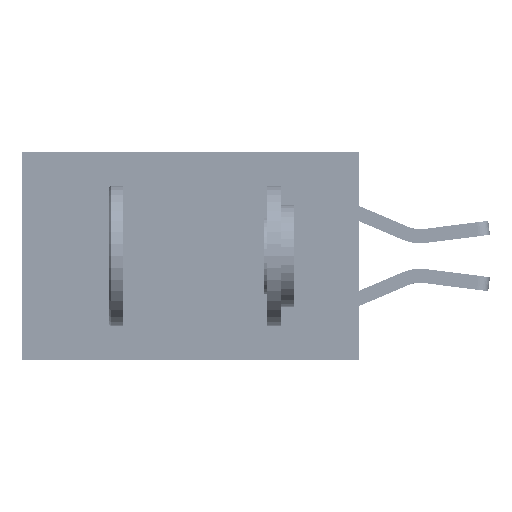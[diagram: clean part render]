
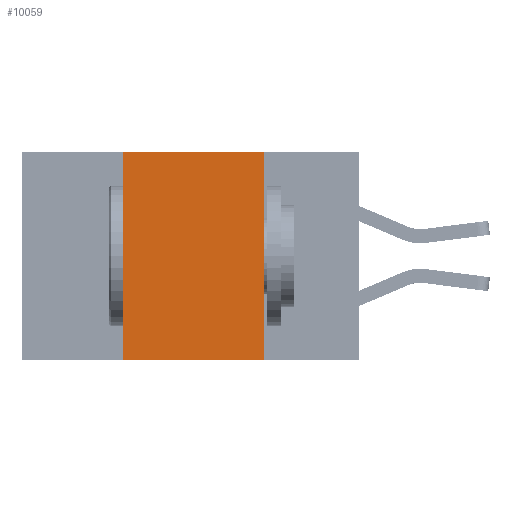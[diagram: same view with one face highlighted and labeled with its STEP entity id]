
A CAD part, left-side view. The second image highlights one B-rep face of the part: STEP entity #10059.
In plain terms, the highlighted planar face has unit normal (-1, 0, 0).
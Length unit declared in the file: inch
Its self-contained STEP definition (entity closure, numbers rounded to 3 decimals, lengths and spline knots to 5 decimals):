
#888 = DIRECTION ( 'NONE',  ( 0., -1., 0. ) ) ;
#1438 = AXIS2_PLACEMENT_3D ( 'NONE', #20532, #17579, #11878 ) ;
#1568 = CARTESIAN_POINT ( 'NONE',  ( 0., 0.17, 0. ) ) ;
#2383 = LINE ( 'NONE', #25675, #35650 ) ;
#6683 = VERTEX_POINT ( 'NONE', #29242 ) ;
#6698 = CARTESIAN_POINT ( 'NONE',  ( 0., 0.17, 0. ) ) ;
#7846 = LINE ( 'NONE', #27850, #27617 ) ;
#10059 = ADVANCED_FACE ( 'NONE', ( #21347 ), #17449, .F. ) ;
#10571 = VECTOR ( 'NONE', #32311, 39.37008 ) ;
#11878 = DIRECTION ( 'NONE',  ( 0., 0., -1. ) ) ;
#11936 = VECTOR ( 'NONE', #23504, 39.37008 ) ;
#13055 = ORIENTED_EDGE ( 'NONE', *, *, #19719, .T. ) ;
#13424 = CARTESIAN_POINT ( 'NONE',  ( 0., 0.6, -0.37 ) ) ;
#17449 = PLANE ( 'NONE',  #1438 ) ;
#17579 = DIRECTION ( 'NONE',  ( 1., 0., 0. ) ) ;
#17670 = ORIENTED_EDGE ( 'NONE', *, *, #34739, .F. ) ;
#18799 = LINE ( 'NONE', #13424, #10571 ) ;
#19719 = EDGE_CURVE ( 'NONE', #39744, #6683, #18799, .T. ) ;
#20236 = EDGE_CURVE ( 'NONE', #22238, #36506, #2383, .T. ) ;
#20532 = CARTESIAN_POINT ( 'NONE',  ( 0., 0.6, 0. ) ) ;
#21257 = ORIENTED_EDGE ( 'NONE', *, *, #36432, .F. ) ;
#21347 = FACE_OUTER_BOUND ( 'NONE', #24152, .T. ) ;
#21725 = ORIENTED_EDGE ( 'NONE', *, *, #20236, .F. ) ;
#22238 = VERTEX_POINT ( 'NONE', #34792 ) ;
#23504 = DIRECTION ( 'NONE',  ( 0., 0., -1. ) ) ;
#24152 = EDGE_LOOP ( 'NONE', ( #17670, #21725, #21257, #13055 ) ) ;
#24487 = DIRECTION ( 'NONE',  ( 0., 0., 1. ) ) ;
#25675 = CARTESIAN_POINT ( 'NONE',  ( 0., 0.6, 0. ) ) ;
#26986 = CARTESIAN_POINT ( 'NONE',  ( 0., 0.42, -0.37 ) ) ;
#27617 = VECTOR ( 'NONE', #24487, 39.37008 ) ;
#27850 = CARTESIAN_POINT ( 'NONE',  ( 0., 0.42, 0. ) ) ;
#29242 = CARTESIAN_POINT ( 'NONE',  ( 0., 0.17, -0.37 ) ) ;
#32311 = DIRECTION ( 'NONE',  ( 0., -1., 0. ) ) ;
#34739 = EDGE_CURVE ( 'NONE', #36506, #6683, #39507, .T. ) ;
#34792 = CARTESIAN_POINT ( 'NONE',  ( 0., 0.42, 0. ) ) ;
#35650 = VECTOR ( 'NONE', #888, 39.37008 ) ;
#36432 = EDGE_CURVE ( 'NONE', #39744, #22238, #7846, .T. ) ;
#36506 = VERTEX_POINT ( 'NONE', #6698 ) ;
#39507 = LINE ( 'NONE', #1568, #11936 ) ;
#39744 = VERTEX_POINT ( 'NONE', #26986 ) ;
